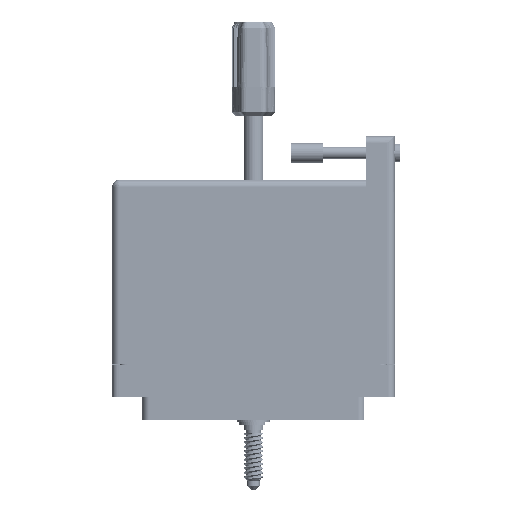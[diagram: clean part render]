
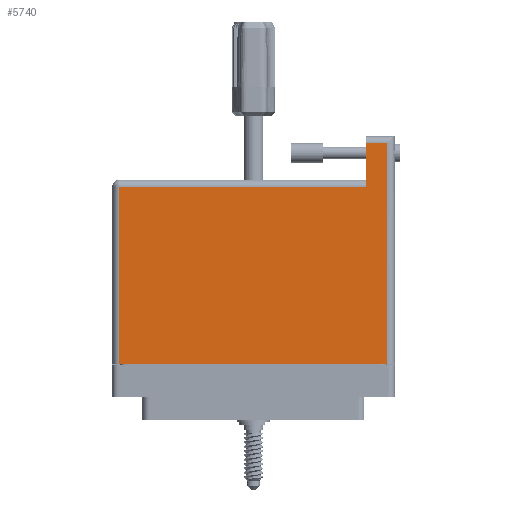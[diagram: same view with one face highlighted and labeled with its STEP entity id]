
A CAD part, front view. The second image highlights one B-rep face of the part: STEP entity #5740.
In plain terms, the highlighted face is planar.
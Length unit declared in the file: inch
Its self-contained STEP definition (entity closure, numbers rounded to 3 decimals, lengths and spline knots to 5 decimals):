
#1507 = DIRECTION ( 'NONE',  ( 1., 0., 0. ) ) ;
#1865 = ORIENTED_EDGE ( 'NONE', *, *, #26630, .T. ) ;
#2381 = DIRECTION ( 'NONE',  ( 0., 1., 0. ) ) ;
#5684 = LINE ( 'NONE', #32305, #21486 ) ;
#5740 = ADVANCED_FACE ( 'NONE', ( #63562 ), #33953, .F. ) ;
#11910 = DIRECTION ( 'NONE',  ( -1., 0., 0. ) ) ;
#12970 = ORIENTED_EDGE ( 'NONE', *, *, #64752, .T. ) ;
#17518 = LINE ( 'NONE', #36776, #61390 ) ;
#17707 = DIRECTION ( 'NONE',  ( 0., -1., 0. ) ) ;
#20232 = DIRECTION ( 'NONE',  ( 0., 0., -1. ) ) ;
#21486 = VECTOR ( 'NONE', #17707, 39.37008 ) ;
#21967 = CARTESIAN_POINT ( 'NONE',  ( 1.079, 1.605, 0.617 ) ) ;
#22373 = LINE ( 'NONE', #51939, #73498 ) ;
#26095 = VERTEX_POINT ( 'NONE', #82649 ) ;
#26630 = EDGE_CURVE ( 'NONE', #50995, #26095, #17518, .T. ) ;
#27807 = LINE ( 'NONE', #49174, #71635 ) ;
#28714 = VECTOR ( 'NONE', #1507, 39.37008 ) ;
#28771 = EDGE_CURVE ( 'NONE', #58416, #65947, #66238, .T. ) ;
#32305 = CARTESIAN_POINT ( 'NONE',  ( -1.289, -0.1, 0.617 ) ) ;
#32699 = VERTEX_POINT ( 'NONE', #60163 ) ;
#33953 = PLANE ( 'NONE',  #78935 ) ;
#36776 = CARTESIAN_POINT ( 'NONE',  ( -1.359, 1.605, 0.617 ) ) ;
#37367 = DIRECTION ( 'NONE',  ( -1., 0., 0. ) ) ;
#39246 = ORIENTED_EDGE ( 'NONE', *, *, #72040, .T. ) ;
#41608 = ORIENTED_EDGE ( 'NONE', *, *, #81020, .T. ) ;
#43047 = DIRECTION ( 'NONE',  ( 0., -1., 0. ) ) ;
#46575 = CARTESIAN_POINT ( 'NONE',  ( -1.289, -0.1, 0.617 ) ) ;
#47519 = CARTESIAN_POINT ( 'NONE',  ( 1.289, -0.1, 0.617 ) ) ;
#48336 = CARTESIAN_POINT ( 'NONE',  ( 1.289, 2.095, 0.617 ) ) ;
#48406 = CARTESIAN_POINT ( 'NONE',  ( 1.289, 2.025, 0.617 ) ) ;
#49174 = CARTESIAN_POINT ( 'NONE',  ( 1.079, 2.095, 0.617 ) ) ;
#50995 = VERTEX_POINT ( 'NONE', #21967 ) ;
#51939 = CARTESIAN_POINT ( 'NONE',  ( -1.359, 2.025, 0.617 ) ) ;
#52110 = EDGE_LOOP ( 'NONE', ( #1865, #41608, #12970, #70244, #58335, #39246 ) ) ;
#55908 = CARTESIAN_POINT ( 'NONE',  ( -1.359, -0.1, 0.617 ) ) ;
#57902 = EDGE_CURVE ( 'NONE', #65947, #32699, #22373, .T. ) ;
#58335 = ORIENTED_EDGE ( 'NONE', *, *, #57902, .T. ) ;
#58416 = VERTEX_POINT ( 'NONE', #47519 ) ;
#60163 = CARTESIAN_POINT ( 'NONE',  ( 1.079, 2.025, 0.617 ) ) ;
#60184 = CARTESIAN_POINT ( 'NONE',  ( -1.359, 1.675, 0.617 ) ) ;
#61390 = VECTOR ( 'NONE', #37367, 39.37008 ) ;
#63562 = FACE_OUTER_BOUND ( 'NONE', #52110, .T. ) ;
#64752 = EDGE_CURVE ( 'NONE', #79451, #58416, #75615, .T. ) ;
#65947 = VERTEX_POINT ( 'NONE', #48406 ) ;
#66238 = LINE ( 'NONE', #48336, #70420 ) ;
#70244 = ORIENTED_EDGE ( 'NONE', *, *, #28771, .T. ) ;
#70420 = VECTOR ( 'NONE', #2381, 39.37008 ) ;
#71635 = VECTOR ( 'NONE', #43047, 39.37008 ) ;
#72040 = EDGE_CURVE ( 'NONE', #32699, #50995, #27807, .T. ) ;
#73498 = VECTOR ( 'NONE', #11910, 39.37008 ) ;
#75615 = LINE ( 'NONE', #55908, #28714 ) ;
#78935 = AXIS2_PLACEMENT_3D ( 'NONE', #60184, #20232, #81200 ) ;
#79451 = VERTEX_POINT ( 'NONE', #46575 ) ;
#81020 = EDGE_CURVE ( 'NONE', #26095, #79451, #5684, .T. ) ;
#81200 = DIRECTION ( 'NONE',  ( -1., 0., 0. ) ) ;
#82649 = CARTESIAN_POINT ( 'NONE',  ( -1.289, 1.605, 0.617 ) ) ;
